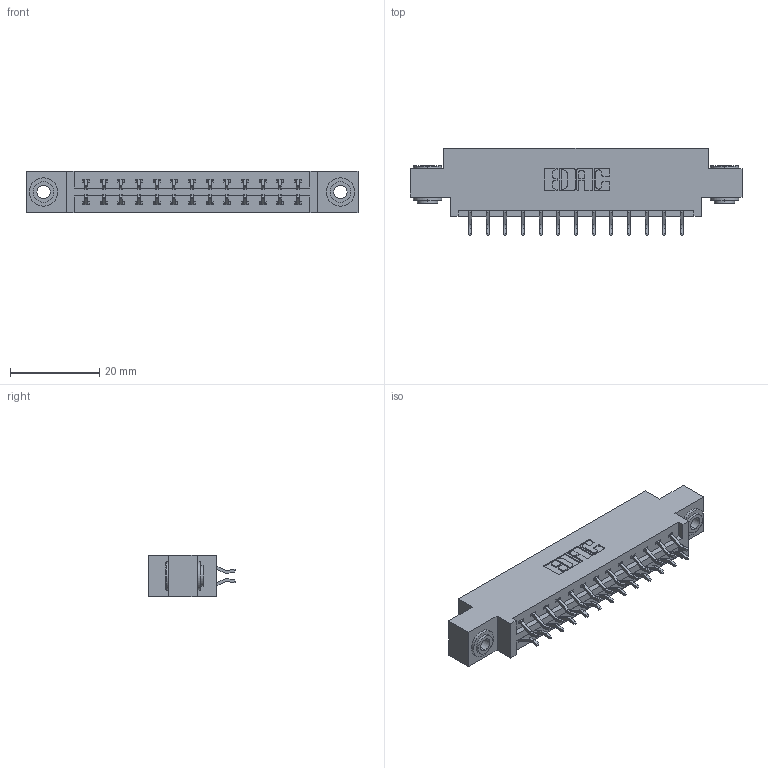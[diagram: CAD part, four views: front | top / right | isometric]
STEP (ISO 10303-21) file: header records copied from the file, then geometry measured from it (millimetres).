
FILE_DESCRIPTION (( 'STEP AP203' ), '1' );
FILE_NAME ('337-026-556-803.STEP', '2019-10-10T22:04:39', ( '' ), ( '' ), 'SwSTEP 2.0', 'SolidWorks 2016', '' );
FILE_SCHEMA (( 'CONFIG_CONTROL_DESIGN' ));
Length unit declared in the file: inch
Products named in the file (4): 337 Part_0.170 Offset - 0.156 Dia-TH; 345-250-002_345-250-002-102; 345-292-001_556 Tail; 337-026-556-803
Assembly tree (29 placements, depth 2):
  337-026-556-803
    337 Part_0.170 Offset - 0.156 Dia-TH
    345-292-001_556 Tail  x26
    345-250-002_345-250-002-102  x2
Bounding box: 74.52 x 19.57 x 9.4 mm (x, y, z)
Volume: 7368.7 mm3; surface area: 8353.5 mm2
Topology: 29 solids, 29 shells, 1716 faces, 5053 edges, 3330 vertices
Faces by surface type: plane 1176, cylinder 532, cone 8
Entity records: 14832 total; most frequent: CARTESIAN_POINT 2513, ORIENTED_EDGE 2430, DIRECTION 2213, EDGE_CURVE 1215, VECTOR 1055, LINE 1055, VERTEX_POINT 806, AXIS2_PLACEMENT_3D 579
